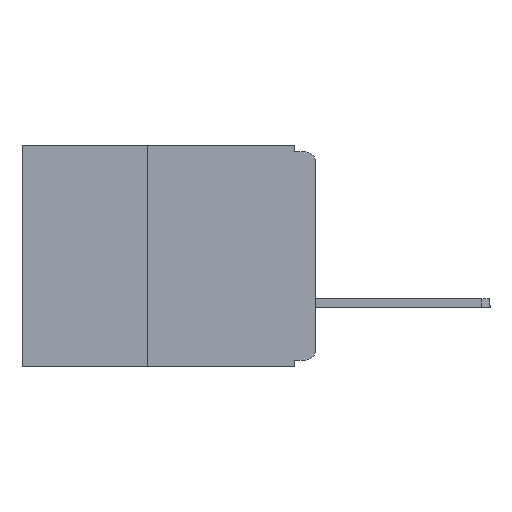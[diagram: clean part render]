
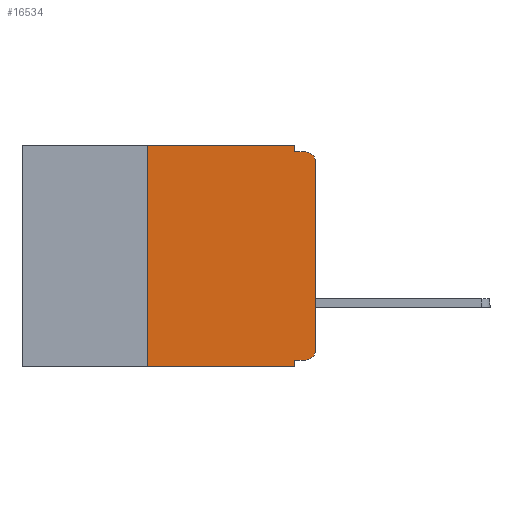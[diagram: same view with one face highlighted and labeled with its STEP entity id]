
A CAD part, left-side view. The second image highlights one B-rep face of the part: STEP entity #16534.
In plain terms, the highlighted planar face has unit normal (-1, 0, 0).
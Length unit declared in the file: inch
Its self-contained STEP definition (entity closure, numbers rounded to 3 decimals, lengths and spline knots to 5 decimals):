
#331 = ORIENTED_EDGE ( 'NONE', *, *, #6632, .T. ) ;
#412 = EDGE_CURVE ( 'NONE', #798, #5506, #5031, .T. ) ;
#579 = CIRCLE ( 'NONE', #12173, 0.015 ) ;
#703 = DIRECTION ( 'NONE',  ( 0., 0., -1. ) ) ;
#798 = VERTEX_POINT ( 'NONE', #8462 ) ;
#884 = LINE ( 'NONE', #5555, #16527 ) ;
#1248 = VECTOR ( 'NONE', #13212, 39.37008 ) ;
#1387 = PLANE ( 'NONE',  #9070 ) ;
#1621 = CARTESIAN_POINT ( 'NONE',  ( 0., 0., 0. ) ) ;
#1809 = ORIENTED_EDGE ( 'NONE', *, *, #2390, .F. ) ;
#2329 = CARTESIAN_POINT ( 'NONE',  ( 0., 0.25, -0.33 ) ) ;
#2390 = EDGE_CURVE ( 'NONE', #11653, #9952, #6569, .T. ) ;
#2754 = CARTESIAN_POINT ( 'NONE',  ( 0., 0.437, 0. ) ) ;
#2796 = CARTESIAN_POINT ( 'NONE',  ( 0., 0.031, 0. ) ) ;
#3295 = FACE_OUTER_BOUND ( 'NONE', #6208, .T. ) ;
#3897 = CARTESIAN_POINT ( 'NONE',  ( 0., 0.031, -0.33 ) ) ;
#4018 = ORIENTED_EDGE ( 'NONE', *, *, #13285, .T. ) ;
#4237 = EDGE_CURVE ( 'NONE', #10721, #9934, #9337, .T. ) ;
#4272 = LINE ( 'NONE', #2754, #12238 ) ;
#4320 = DIRECTION ( 'NONE',  ( 0., -1., 0. ) ) ;
#4370 = DIRECTION ( 'NONE',  ( 0., 0., -1. ) ) ;
#5031 = CIRCLE ( 'NONE', #5891, 0.015 ) ;
#5401 = DIRECTION ( 'NONE',  ( 0., 0., -1. ) ) ;
#5449 = DIRECTION ( 'NONE',  ( -1., 0., 0. ) ) ;
#5468 = ORIENTED_EDGE ( 'NONE', *, *, #8515, .F. ) ;
#5476 = CARTESIAN_POINT ( 'NONE',  ( 0., 0.015, -0.025 ) ) ;
#5506 = VERTEX_POINT ( 'NONE', #16099 ) ;
#5555 = CARTESIAN_POINT ( 'NONE',  ( 0., 0., -0.32 ) ) ;
#5565 = VERTEX_POINT ( 'NONE', #15283 ) ;
#5743 = CARTESIAN_POINT ( 'NONE',  ( 0., 0.031, -0.01 ) ) ;
#5891 = AXIS2_PLACEMENT_3D ( 'NONE', #16358, #15493, #703 ) ;
#6029 = DIRECTION ( 'NONE',  ( 0., 0., -1. ) ) ;
#6208 = EDGE_LOOP ( 'NONE', ( #4018, #331, #8509, #16480, #8976, #5468, #17410, #1809, #13890, #17905 ) ) ;
#6256 = DIRECTION ( 'NONE',  ( 0., 0., 1. ) ) ;
#6481 = EDGE_CURVE ( 'NONE', #16939, #9952, #7589, .T. ) ;
#6569 = LINE ( 'NONE', #13733, #18514 ) ;
#6632 = EDGE_CURVE ( 'NONE', #16068, #9934, #579, .T. ) ;
#7042 = CARTESIAN_POINT ( 'NONE',  ( 0., 0.437, -0.33 ) ) ;
#7045 = DIRECTION ( 'NONE',  ( 0., -1., 0. ) ) ;
#7589 = LINE ( 'NONE', #7042, #15533 ) ;
#8462 = CARTESIAN_POINT ( 'NONE',  ( 0., 0.015, -0.32 ) ) ;
#8496 = CARTESIAN_POINT ( 'NONE',  ( 0., 0.015, -0.01 ) ) ;
#8509 = ORIENTED_EDGE ( 'NONE', *, *, #4237, .F. ) ;
#8515 = EDGE_CURVE ( 'NONE', #16939, #5565, #10030, .T. ) ;
#8919 = CARTESIAN_POINT ( 'NONE',  ( 0., 0.437, 0. ) ) ;
#8976 = ORIENTED_EDGE ( 'NONE', *, *, #16458, .F. ) ;
#9070 = AXIS2_PLACEMENT_3D ( 'NONE', #8919, #14982, #6029 ) ;
#9337 = LINE ( 'NONE', #13006, #1248 ) ;
#9482 = EDGE_CURVE ( 'NONE', #15360, #10721, #11432, .T. ) ;
#9612 = VECTOR ( 'NONE', #6256, 39.37008 ) ;
#9675 = CARTESIAN_POINT ( 'NONE',  ( 0., 0.031, -0.32 ) ) ;
#9934 = VERTEX_POINT ( 'NONE', #8496 ) ;
#9952 = VERTEX_POINT ( 'NONE', #3897 ) ;
#9965 = CARTESIAN_POINT ( 'NONE',  ( 0., 0.031, 0. ) ) ;
#10030 = LINE ( 'NONE', #13965, #14031 ) ;
#10643 = EDGE_CURVE ( 'NONE', #798, #11653, #884, .T. ) ;
#10721 = VERTEX_POINT ( 'NONE', #5743 ) ;
#10874 = CARTESIAN_POINT ( 'NONE',  ( 0., 0., -0.025 ) ) ;
#11432 = LINE ( 'NONE', #2796, #19385 ) ;
#11653 = VERTEX_POINT ( 'NONE', #9675 ) ;
#12173 = AXIS2_PLACEMENT_3D ( 'NONE', #5476, #5449, #5401 ) ;
#12238 = VECTOR ( 'NONE', #4320, 39.37008 ) ;
#13006 = CARTESIAN_POINT ( 'NONE',  ( 0., 0., -0.01 ) ) ;
#13212 = DIRECTION ( 'NONE',  ( 0., -1., 0. ) ) ;
#13285 = EDGE_CURVE ( 'NONE', #5506, #16068, #13620, .T. ) ;
#13620 = LINE ( 'NONE', #1621, #9612 ) ;
#13733 = CARTESIAN_POINT ( 'NONE',  ( 0., 0.031, -0.33 ) ) ;
#13740 = DIRECTION ( 'NONE',  ( 0., 0., -1. ) ) ;
#13890 = ORIENTED_EDGE ( 'NONE', *, *, #10643, .F. ) ;
#13965 = CARTESIAN_POINT ( 'NONE',  ( 0., 0.25, -0.33 ) ) ;
#14031 = VECTOR ( 'NONE', #16985, 39.37008 ) ;
#14982 = DIRECTION ( 'NONE',  ( 1., 0., 0. ) ) ;
#15283 = CARTESIAN_POINT ( 'NONE',  ( 0., 0.25, 0. ) ) ;
#15360 = VERTEX_POINT ( 'NONE', #9965 ) ;
#15493 = DIRECTION ( 'NONE',  ( -1., 0., 0. ) ) ;
#15533 = VECTOR ( 'NONE', #7045, 39.37008 ) ;
#16068 = VERTEX_POINT ( 'NONE', #10874 ) ;
#16099 = CARTESIAN_POINT ( 'NONE',  ( 0., 0., -0.305 ) ) ;
#16358 = CARTESIAN_POINT ( 'NONE',  ( 0., 0.015, -0.305 ) ) ;
#16458 = EDGE_CURVE ( 'NONE', #5565, #15360, #4272, .T. ) ;
#16480 = ORIENTED_EDGE ( 'NONE', *, *, #9482, .F. ) ;
#16527 = VECTOR ( 'NONE', #19007, 39.37008 ) ;
#16534 = ADVANCED_FACE ( 'NONE', ( #3295 ), #1387, .F. ) ;
#16939 = VERTEX_POINT ( 'NONE', #2329 ) ;
#16985 = DIRECTION ( 'NONE',  ( 0., 0., 1. ) ) ;
#17410 = ORIENTED_EDGE ( 'NONE', *, *, #6481, .T. ) ;
#17905 = ORIENTED_EDGE ( 'NONE', *, *, #412, .T. ) ;
#18514 = VECTOR ( 'NONE', #13740, 39.37008 ) ;
#19007 = DIRECTION ( 'NONE',  ( 0., 1., 0. ) ) ;
#19385 = VECTOR ( 'NONE', #4370, 39.37008 ) ;
